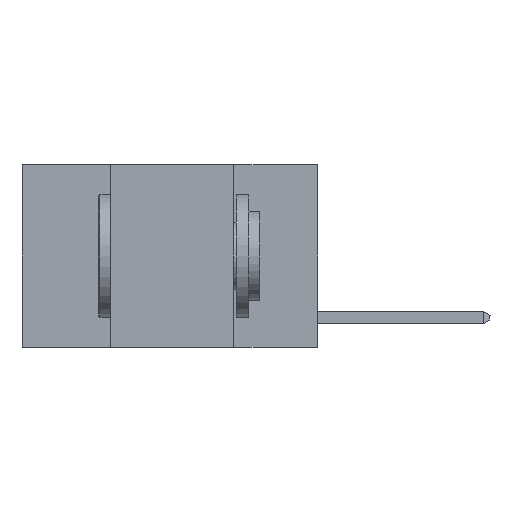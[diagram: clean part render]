
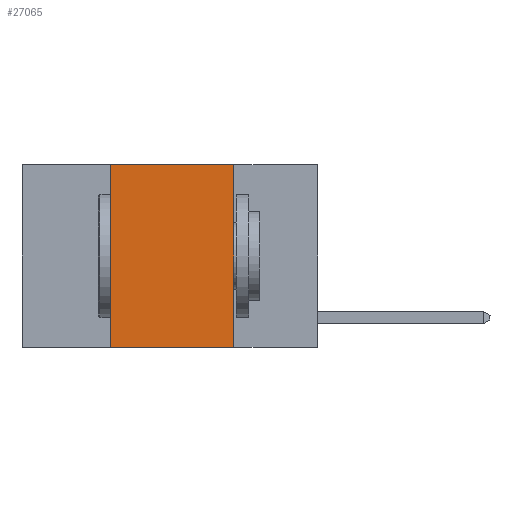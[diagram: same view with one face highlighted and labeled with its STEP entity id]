
A CAD part, left-side view. The second image highlights one B-rep face of the part: STEP entity #27065.
In plain terms, the highlighted planar face has unit normal (-1, 0, 0).
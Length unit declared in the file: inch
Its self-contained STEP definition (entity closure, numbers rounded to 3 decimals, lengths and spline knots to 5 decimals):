
#1674 = EDGE_CURVE ( 'NONE', #8809, #10663, #2723, .T. ) ;
#2124 = VERTEX_POINT ( 'NONE', #8140 ) ;
#2480 = CARTESIAN_POINT ( 'NONE',  ( 0., 0.6, 0. ) ) ;
#2723 = LINE ( 'NONE', #5840, #23166 ) ;
#5028 = CARTESIAN_POINT ( 'NONE',  ( 0., 0.42, 0. ) ) ;
#5085 = EDGE_CURVE ( 'NONE', #18609, #10663, #11243, .T. ) ;
#5840 = CARTESIAN_POINT ( 'NONE',  ( 0., 0.17, 0. ) ) ;
#6463 = DIRECTION ( 'NONE',  ( 0., 0., -1. ) ) ;
#6905 = DIRECTION ( 'NONE',  ( 1., 0., 0. ) ) ;
#8140 = CARTESIAN_POINT ( 'NONE',  ( 0., 0.42, 0. ) ) ;
#8809 = VERTEX_POINT ( 'NONE', #13538 ) ;
#9857 = ORIENTED_EDGE ( 'NONE', *, *, #23979, .F. ) ;
#9994 = VECTOR ( 'NONE', #19782, 39.37008 ) ;
#10351 = ORIENTED_EDGE ( 'NONE', *, *, #1674, .F. ) ;
#10663 = VERTEX_POINT ( 'NONE', #19837 ) ;
#11108 = ORIENTED_EDGE ( 'NONE', *, *, #5085, .T. ) ;
#11243 = LINE ( 'NONE', #17933, #22178 ) ;
#11776 = EDGE_LOOP ( 'NONE', ( #10351, #9857, #13976, #11108 ) ) ;
#12032 = DIRECTION ( 'NONE',  ( 0., -1., 0. ) ) ;
#13021 = PLANE ( 'NONE',  #25493 ) ;
#13538 = CARTESIAN_POINT ( 'NONE',  ( 0., 0.17, 0. ) ) ;
#13976 = ORIENTED_EDGE ( 'NONE', *, *, #17743, .F. ) ;
#14415 = LINE ( 'NONE', #20484, #24703 ) ;
#15294 = LINE ( 'NONE', #5028, #9994 ) ;
#17743 = EDGE_CURVE ( 'NONE', #18609, #2124, #15294, .T. ) ;
#17933 = CARTESIAN_POINT ( 'NONE',  ( 0., 0.6, -0.37 ) ) ;
#18511 = FACE_OUTER_BOUND ( 'NONE', #11776, .T. ) ;
#18609 = VERTEX_POINT ( 'NONE', #24578 ) ;
#19782 = DIRECTION ( 'NONE',  ( 0., 0., 1. ) ) ;
#19837 = CARTESIAN_POINT ( 'NONE',  ( 0., 0.17, -0.37 ) ) ;
#20080 = DIRECTION ( 'NONE',  ( 0., -1., 0. ) ) ;
#20484 = CARTESIAN_POINT ( 'NONE',  ( 0., 0.6, 0. ) ) ;
#22178 = VECTOR ( 'NONE', #20080, 39.37008 ) ;
#23166 = VECTOR ( 'NONE', #6463, 39.37008 ) ;
#23405 = DIRECTION ( 'NONE',  ( 0., 0., -1. ) ) ;
#23979 = EDGE_CURVE ( 'NONE', #2124, #8809, #14415, .T. ) ;
#24578 = CARTESIAN_POINT ( 'NONE',  ( 0., 0.42, -0.37 ) ) ;
#24703 = VECTOR ( 'NONE', #12032, 39.37008 ) ;
#25493 = AXIS2_PLACEMENT_3D ( 'NONE', #2480, #6905, #23405 ) ;
#27065 = ADVANCED_FACE ( 'NONE', ( #18511 ), #13021, .F. ) ;
